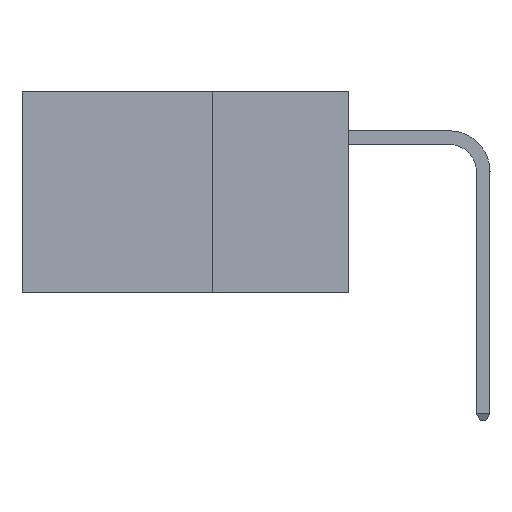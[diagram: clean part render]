
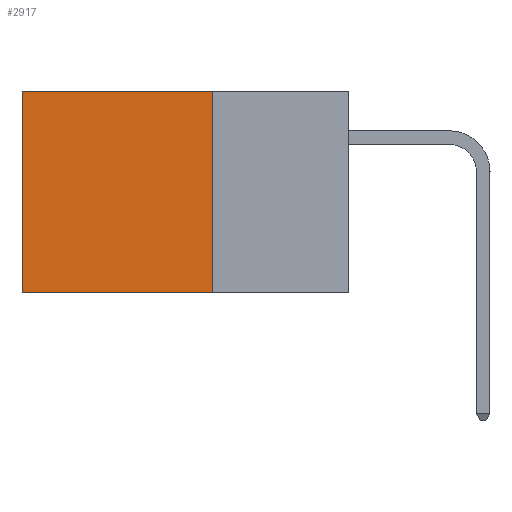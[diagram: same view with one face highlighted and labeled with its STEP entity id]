
A CAD part, left-side view. The second image highlights one B-rep face of the part: STEP entity #2917.
In plain terms, the highlighted planar face has unit normal (-1, 0, 0).
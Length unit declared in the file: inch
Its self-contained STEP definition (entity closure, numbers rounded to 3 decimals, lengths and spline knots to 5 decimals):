
#803 = CARTESIAN_POINT ( 'NONE',  ( 0.2875, 0.25, 0. ) ) ;
#2576 = VECTOR ( 'NONE', #3015, 39.37008 ) ;
#2909 = CARTESIAN_POINT ( 'NONE',  ( 0.2875, 0.25, 0. ) ) ;
#2917 = ADVANCED_FACE ( 'NONE', ( #4010 ), #35143, .F. ) ;
#3015 = DIRECTION ( 'NONE',  ( 0., 1., 0. ) ) ;
#3177 = CARTESIAN_POINT ( 'NONE',  ( 0.2875, 0.25, -0.37 ) ) ;
#4010 = FACE_OUTER_BOUND ( 'NONE', #35163, .T. ) ;
#4178 = DIRECTION ( 'NONE',  ( 0., 0., -1. ) ) ;
#4448 = EDGE_CURVE ( 'NONE', #10714, #28226, #9089, .T. ) ;
#4488 = ORIENTED_EDGE ( 'NONE', *, *, #4448, .F. ) ;
#6772 = CARTESIAN_POINT ( 'NONE',  ( 0.2875, 0.6, 0. ) ) ;
#8079 = CARTESIAN_POINT ( 'NONE',  ( 0.2875, 0.25, 0. ) ) ;
#9089 = LINE ( 'NONE', #3177, #2576 ) ;
#9216 = LINE ( 'NONE', #2909, #15676 ) ;
#10714 = VERTEX_POINT ( 'NONE', #31604 ) ;
#13269 = EDGE_CURVE ( 'NONE', #29377, #28226, #29196, .T. ) ;
#13792 = VECTOR ( 'NONE', #28747, 39.37008 ) ;
#15676 = VECTOR ( 'NONE', #32994, 39.37008 ) ;
#15772 = EDGE_CURVE ( 'NONE', #28510, #29377, #9216, .T. ) ;
#17107 = EDGE_CURVE ( 'NONE', #28510, #10714, #22953, .T. ) ;
#18331 = ORIENTED_EDGE ( 'NONE', *, *, #15772, .T. ) ;
#19031 = AXIS2_PLACEMENT_3D ( 'NONE', #803, #35075, #34981 ) ;
#22706 = ORIENTED_EDGE ( 'NONE', *, *, #17107, .F. ) ;
#22953 = LINE ( 'NONE', #34050, #29264 ) ;
#26066 = CARTESIAN_POINT ( 'NONE',  ( 0.2875, 0.6, -0.37 ) ) ;
#26112 = CARTESIAN_POINT ( 'NONE',  ( 0.2875, 0.6, 0. ) ) ;
#28226 = VERTEX_POINT ( 'NONE', #26066 ) ;
#28510 = VERTEX_POINT ( 'NONE', #8079 ) ;
#28747 = DIRECTION ( 'NONE',  ( 0., 0., -1. ) ) ;
#29196 = LINE ( 'NONE', #6772, #13792 ) ;
#29264 = VECTOR ( 'NONE', #4178, 39.37008 ) ;
#29377 = VERTEX_POINT ( 'NONE', #26112 ) ;
#31604 = CARTESIAN_POINT ( 'NONE',  ( 0.2875, 0.25, -0.37 ) ) ;
#32538 = ORIENTED_EDGE ( 'NONE', *, *, #13269, .T. ) ;
#32994 = DIRECTION ( 'NONE',  ( 0., 1., 0. ) ) ;
#34050 = CARTESIAN_POINT ( 'NONE',  ( 0.2875, 0.25, 0. ) ) ;
#34981 = DIRECTION ( 'NONE',  ( 0., 0., -1. ) ) ;
#35075 = DIRECTION ( 'NONE',  ( 1., 0., 0. ) ) ;
#35143 = PLANE ( 'NONE',  #19031 ) ;
#35163 = EDGE_LOOP ( 'NONE', ( #32538, #4488, #22706, #18331 ) ) ;
